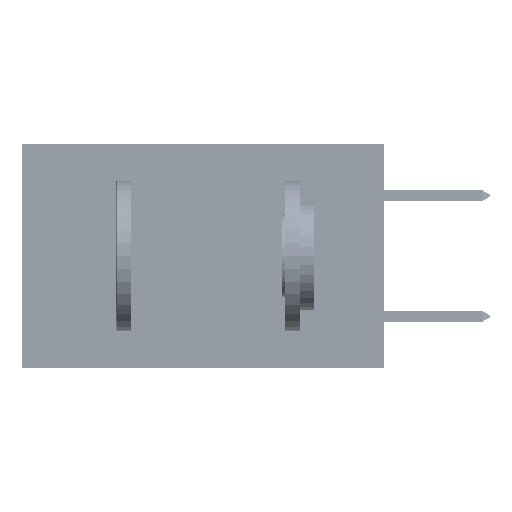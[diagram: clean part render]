
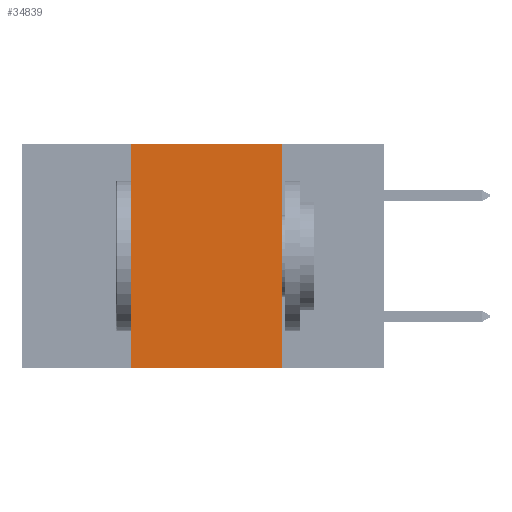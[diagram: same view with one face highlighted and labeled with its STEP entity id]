
A CAD part, left-side view. The second image highlights one B-rep face of the part: STEP entity #34839.
In plain terms, the highlighted planar face has unit normal (-1, 0, 0).
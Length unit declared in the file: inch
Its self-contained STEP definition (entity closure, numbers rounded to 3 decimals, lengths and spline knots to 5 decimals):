
#3691 = FACE_OUTER_BOUND ( 'NONE', #43127, .T. ) ;
#5196 = VERTEX_POINT ( 'NONE', #30588 ) ;
#5446 = PLANE ( 'NONE',  #22016 ) ;
#7206 = ORIENTED_EDGE ( 'NONE', *, *, #21367, .F. ) ;
#7314 = LINE ( 'NONE', #41672, #21823 ) ;
#7343 = VECTOR ( 'NONE', #37657, 39.37008 ) ;
#8286 = VERTEX_POINT ( 'NONE', #30164 ) ;
#9157 = EDGE_CURVE ( 'NONE', #38477, #8286, #26416, .T. ) ;
#11465 = DIRECTION ( 'NONE',  ( 0., -1., 0. ) ) ;
#12904 = EDGE_CURVE ( 'NONE', #41031, #8286, #43607, .T. ) ;
#16869 = LINE ( 'NONE', #19564, #7343 ) ;
#19564 = CARTESIAN_POINT ( 'NONE',  ( 0., 0.42, 0. ) ) ;
#20456 = CARTESIAN_POINT ( 'NONE',  ( 0., 0.17, 0. ) ) ;
#20901 = ORIENTED_EDGE ( 'NONE', *, *, #9157, .F. ) ;
#21367 = EDGE_CURVE ( 'NONE', #41031, #5196, #16869, .T. ) ;
#21823 = VECTOR ( 'NONE', #41375, 39.37008 ) ;
#22016 = AXIS2_PLACEMENT_3D ( 'NONE', #30284, #40910, #26991 ) ;
#22188 = ORIENTED_EDGE ( 'NONE', *, *, #42532, .F. ) ;
#25927 = CARTESIAN_POINT ( 'NONE',  ( 0., 0.6, -0.37 ) ) ;
#26416 = LINE ( 'NONE', #20456, #38720 ) ;
#26991 = DIRECTION ( 'NONE',  ( 0., 0., -1. ) ) ;
#30164 = CARTESIAN_POINT ( 'NONE',  ( 0., 0.17, -0.37 ) ) ;
#30284 = CARTESIAN_POINT ( 'NONE',  ( 0., 0.6, 0. ) ) ;
#30588 = CARTESIAN_POINT ( 'NONE',  ( 0., 0.42, 0. ) ) ;
#34143 = VECTOR ( 'NONE', #11465, 39.37008 ) ;
#34807 = CARTESIAN_POINT ( 'NONE',  ( 0., 0.17, 0. ) ) ;
#34839 = ADVANCED_FACE ( 'NONE', ( #3691 ), #5446, .F. ) ;
#35270 = DIRECTION ( 'NONE',  ( 0., 0., -1. ) ) ;
#37657 = DIRECTION ( 'NONE',  ( 0., 0., 1. ) ) ;
#38477 = VERTEX_POINT ( 'NONE', #34807 ) ;
#38720 = VECTOR ( 'NONE', #35270, 39.37008 ) ;
#40910 = DIRECTION ( 'NONE',  ( 1., 0., 0. ) ) ;
#41031 = VERTEX_POINT ( 'NONE', #45865 ) ;
#41375 = DIRECTION ( 'NONE',  ( 0., -1., 0. ) ) ;
#41672 = CARTESIAN_POINT ( 'NONE',  ( 0., 0.6, 0. ) ) ;
#42532 = EDGE_CURVE ( 'NONE', #5196, #38477, #7314, .T. ) ;
#42663 = ORIENTED_EDGE ( 'NONE', *, *, #12904, .T. ) ;
#43127 = EDGE_LOOP ( 'NONE', ( #20901, #22188, #7206, #42663 ) ) ;
#43607 = LINE ( 'NONE', #25927, #34143 ) ;
#45865 = CARTESIAN_POINT ( 'NONE',  ( 0., 0.42, -0.37 ) ) ;
